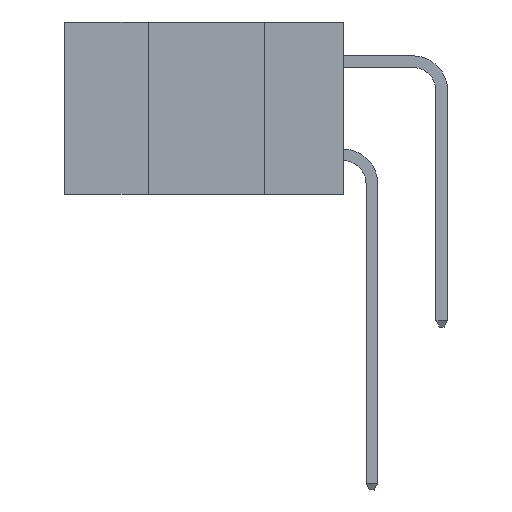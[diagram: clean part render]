
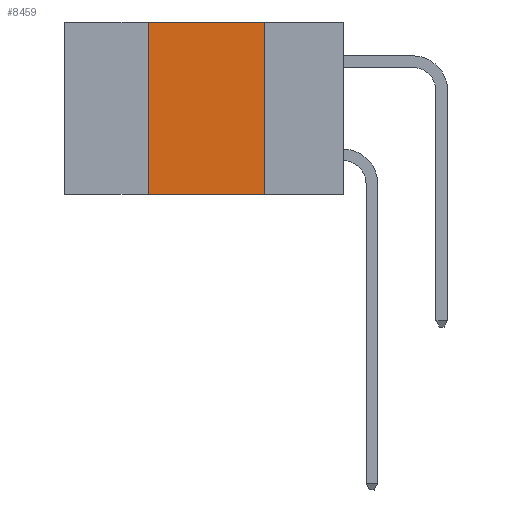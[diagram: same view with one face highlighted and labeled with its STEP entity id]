
A CAD part, left-side view. The second image highlights one B-rep face of the part: STEP entity #8459.
In plain terms, the highlighted planar face has unit normal (-1, 0, 0).
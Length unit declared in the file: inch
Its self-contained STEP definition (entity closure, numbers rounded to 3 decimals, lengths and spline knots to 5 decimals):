
#69 = ORIENTED_EDGE ( 'NONE', *, *, #10290, .F. ) ;
#257 = DIRECTION ( 'NONE',  ( 1., 0., 0. ) ) ;
#798 = EDGE_CURVE ( 'NONE', #11270, #8984, #9080, .T. ) ;
#1242 = LINE ( 'NONE', #13036, #9474 ) ;
#1393 = VERTEX_POINT ( 'NONE', #12742 ) ;
#1516 = CARTESIAN_POINT ( 'NONE',  ( 0., 0.42, 0. ) ) ;
#1717 = ORIENTED_EDGE ( 'NONE', *, *, #8534, .T. ) ;
#1852 = CARTESIAN_POINT ( 'NONE',  ( 0., 0.17, 0. ) ) ;
#1863 = VERTEX_POINT ( 'NONE', #8753 ) ;
#3033 = LINE ( 'NONE', #1852, #6251 ) ;
#4264 = ORIENTED_EDGE ( 'NONE', *, *, #798, .F. ) ;
#4488 = CARTESIAN_POINT ( 'NONE',  ( 0., 0.42, -0.37 ) ) ;
#6248 = VECTOR ( 'NONE', #11032, 39.37008 ) ;
#6251 = VECTOR ( 'NONE', #11503, 39.37008 ) ;
#6321 = DIRECTION ( 'NONE',  ( 0., -1., 0. ) ) ;
#7246 = DIRECTION ( 'NONE',  ( 0., -1., 0. ) ) ;
#7610 = FACE_OUTER_BOUND ( 'NONE', #11724, .T. ) ;
#8052 = DIRECTION ( 'NONE',  ( 0., 0., -1. ) ) ;
#8459 = ADVANCED_FACE ( 'NONE', ( #7610 ), #12606, .F. ) ;
#8534 = EDGE_CURVE ( 'NONE', #11270, #1393, #1242, .T. ) ;
#8753 = CARTESIAN_POINT ( 'NONE',  ( 0., 0.17, 0. ) ) ;
#8949 = VECTOR ( 'NONE', #6321, 39.37008 ) ;
#8984 = VERTEX_POINT ( 'NONE', #1516 ) ;
#9080 = LINE ( 'NONE', #10700, #6248 ) ;
#9245 = EDGE_CURVE ( 'NONE', #8984, #1863, #12135, .T. ) ;
#9474 = VECTOR ( 'NONE', #7246, 39.37008 ) ;
#9488 = CARTESIAN_POINT ( 'NONE',  ( 0., 0.6, 0. ) ) ;
#10290 = EDGE_CURVE ( 'NONE', #1863, #1393, #3033, .T. ) ;
#10307 = AXIS2_PLACEMENT_3D ( 'NONE', #11665, #257, #8052 ) ;
#10700 = CARTESIAN_POINT ( 'NONE',  ( 0., 0.42, 0. ) ) ;
#11032 = DIRECTION ( 'NONE',  ( 0., 0., 1. ) ) ;
#11270 = VERTEX_POINT ( 'NONE', #4488 ) ;
#11433 = ORIENTED_EDGE ( 'NONE', *, *, #9245, .F. ) ;
#11503 = DIRECTION ( 'NONE',  ( 0., 0., -1. ) ) ;
#11665 = CARTESIAN_POINT ( 'NONE',  ( 0., 0.6, 0. ) ) ;
#11724 = EDGE_LOOP ( 'NONE', ( #69, #11433, #4264, #1717 ) ) ;
#12135 = LINE ( 'NONE', #9488, #8949 ) ;
#12606 = PLANE ( 'NONE',  #10307 ) ;
#12742 = CARTESIAN_POINT ( 'NONE',  ( 0., 0.17, -0.37 ) ) ;
#13036 = CARTESIAN_POINT ( 'NONE',  ( 0., 0.6, -0.37 ) ) ;
